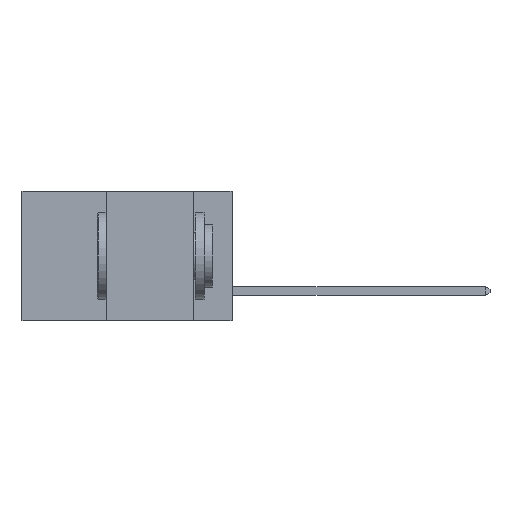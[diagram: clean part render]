
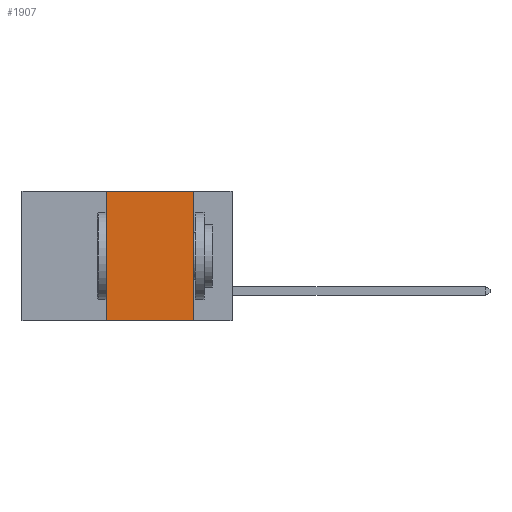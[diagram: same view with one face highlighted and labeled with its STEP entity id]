
A CAD part, left-side view. The second image highlights one B-rep face of the part: STEP entity #1907.
In plain terms, the highlighted planar face has unit normal (-1, 0, 0).
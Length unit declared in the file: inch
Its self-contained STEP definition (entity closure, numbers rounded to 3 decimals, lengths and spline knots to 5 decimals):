
#125 = DIRECTION ( 'NONE',  ( 0., -1., 0. ) ) ;
#773 = VERTEX_POINT ( 'NONE', #7982 ) ;
#1783 = CARTESIAN_POINT ( 'NONE',  ( 0., 0.11, 0. ) ) ;
#1907 = ADVANCED_FACE ( 'NONE', ( #10394 ), #12446, .F. ) ;
#2131 = VECTOR ( 'NONE', #10149, 39.37008 ) ;
#2146 = EDGE_CURVE ( 'NONE', #7780, #3033, #7626, .T. ) ;
#2429 = CARTESIAN_POINT ( 'NONE',  ( 0., 0.11, 0. ) ) ;
#3033 = VERTEX_POINT ( 'NONE', #2429 ) ;
#3151 = VECTOR ( 'NONE', #4962, 39.37008 ) ;
#3493 = LINE ( 'NONE', #11263, #5279 ) ;
#4285 = EDGE_LOOP ( 'NONE', ( #4800, #7804, #12974, #10736 ) ) ;
#4800 = ORIENTED_EDGE ( 'NONE', *, *, #9088, .F. ) ;
#4962 = DIRECTION ( 'NONE',  ( 0., 0., -1. ) ) ;
#5279 = VECTOR ( 'NONE', #125, 39.37008 ) ;
#5507 = LINE ( 'NONE', #7958, #8159 ) ;
#5592 = CARTESIAN_POINT ( 'NONE',  ( 0., 0.36, -0.37 ) ) ;
#5909 = LINE ( 'NONE', #1783, #3151 ) ;
#7626 = LINE ( 'NONE', #10200, #2131 ) ;
#7780 = VERTEX_POINT ( 'NONE', #12835 ) ;
#7804 = ORIENTED_EDGE ( 'NONE', *, *, #2146, .F. ) ;
#7958 = CARTESIAN_POINT ( 'NONE',  ( 0., 0.36, 0. ) ) ;
#7982 = CARTESIAN_POINT ( 'NONE',  ( 0., 0.11, -0.37 ) ) ;
#8159 = VECTOR ( 'NONE', #12810, 39.37008 ) ;
#8662 = EDGE_CURVE ( 'NONE', #12280, #773, #3493, .T. ) ;
#8727 = AXIS2_PLACEMENT_3D ( 'NONE', #12426, #12370, #12345 ) ;
#9088 = EDGE_CURVE ( 'NONE', #3033, #773, #5909, .T. ) ;
#10149 = DIRECTION ( 'NONE',  ( 0., -1., 0. ) ) ;
#10200 = CARTESIAN_POINT ( 'NONE',  ( 0., 0.6, 0. ) ) ;
#10394 = FACE_OUTER_BOUND ( 'NONE', #4285, .T. ) ;
#10736 = ORIENTED_EDGE ( 'NONE', *, *, #8662, .T. ) ;
#11263 = CARTESIAN_POINT ( 'NONE',  ( 0., 0.6, -0.37 ) ) ;
#11990 = EDGE_CURVE ( 'NONE', #12280, #7780, #5507, .T. ) ;
#12280 = VERTEX_POINT ( 'NONE', #5592 ) ;
#12345 = DIRECTION ( 'NONE',  ( 0., 0., -1. ) ) ;
#12370 = DIRECTION ( 'NONE',  ( 1., 0., 0. ) ) ;
#12426 = CARTESIAN_POINT ( 'NONE',  ( 0., 0.6, 0. ) ) ;
#12446 = PLANE ( 'NONE',  #8727 ) ;
#12810 = DIRECTION ( 'NONE',  ( 0., 0., 1. ) ) ;
#12835 = CARTESIAN_POINT ( 'NONE',  ( 0., 0.36, 0. ) ) ;
#12974 = ORIENTED_EDGE ( 'NONE', *, *, #11990, .F. ) ;
